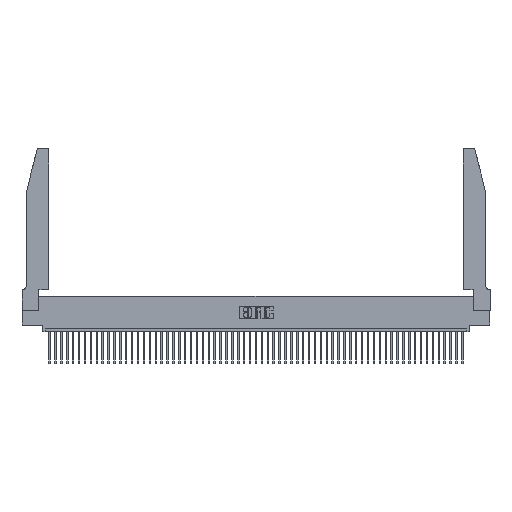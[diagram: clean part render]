
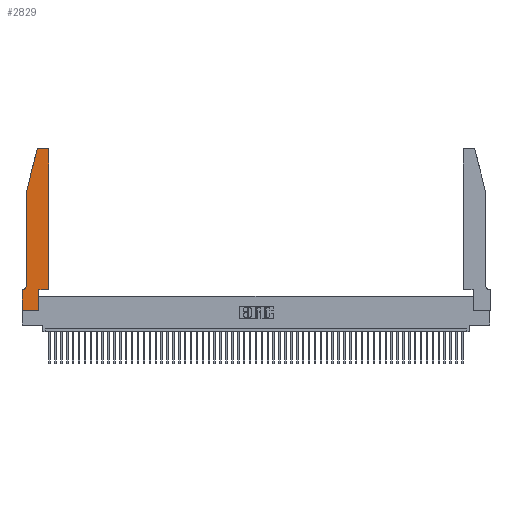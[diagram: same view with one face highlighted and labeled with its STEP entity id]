
A CAD part, top view. The second image highlights one B-rep face of the part: STEP entity #2829.
In plain terms, the highlighted planar face has unit normal (0, 0, 1).
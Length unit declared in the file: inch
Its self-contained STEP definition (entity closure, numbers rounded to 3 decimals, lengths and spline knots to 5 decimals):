
#566 = EDGE_CURVE ( 'NONE', #36919, #50856, #39967, .T. ) ;
#1370 = CARTESIAN_POINT ( 'NONE',  ( 0.284, 2.72, 0.37 ) ) ;
#1416 = CARTESIAN_POINT ( 'NONE',  ( 0.2865, 0.35, 0.37 ) ) ;
#1967 = VERTEX_POINT ( 'NONE', #28017 ) ;
#2055 = DIRECTION ( 'NONE',  ( 0., 0., 1. ) ) ;
#2248 = ORIENTED_EDGE ( 'NONE', *, *, #53547, .T. ) ;
#2305 = DIRECTION ( 'NONE',  ( 0., 1., 0. ) ) ;
#2829 = ADVANCED_FACE ( 'NONE', ( #20331 ), #9238, .T. ) ;
#3087 = EDGE_CURVE ( 'NONE', #14499, #12628, #45249, .T. ) ;
#3220 = CARTESIAN_POINT ( 'NONE',  ( 0.0755, 0.35, 0.37 ) ) ;
#4333 = CARTESIAN_POINT ( 'NONE',  ( 0.4505, 0.35, 0.37 ) ) ;
#5033 = VECTOR ( 'NONE', #30025, 39.37008 ) ;
#5666 = VERTEX_POINT ( 'NONE', #31880 ) ;
#5873 = LINE ( 'NONE', #32470, #36101 ) ;
#6248 = LINE ( 'NONE', #3220, #34407 ) ;
#7777 = AXIS2_PLACEMENT_3D ( 'NONE', #36329, #44796, #54358 ) ;
#8421 = AXIS2_PLACEMENT_3D ( 'NONE', #1370, #13735, #34801 ) ;
#8667 = CARTESIAN_POINT ( 'NONE',  ( 0.0055, 0.35, 0.37 ) ) ;
#8744 = ORIENTED_EDGE ( 'NONE', *, *, #42962, .T. ) ;
#9056 = DIRECTION ( 'NONE',  ( -0.239, -0.971, 0. ) ) ;
#9238 = PLANE ( 'NONE',  #32448 ) ;
#9537 = CIRCLE ( 'NONE', #7777, 0.07 ) ;
#9663 = VECTOR ( 'NONE', #33040, 39.37008 ) ;
#12628 = VERTEX_POINT ( 'NONE', #13793 ) ;
#13256 = CARTESIAN_POINT ( 'NONE',  ( 0.0755, 0.42, 0.37 ) ) ;
#13407 = DIRECTION ( 'NONE',  ( 0., 0., 1. ) ) ;
#13735 = DIRECTION ( 'NONE',  ( 0., 0., 1. ) ) ;
#13793 = CARTESIAN_POINT ( 'NONE',  ( 0.2865, 0., 0.37 ) ) ;
#14499 = VERTEX_POINT ( 'NONE', #18149 ) ;
#15003 = VERTEX_POINT ( 'NONE', #18124 ) ;
#16359 = VECTOR ( 'NONE', #44993, 39.37008 ) ;
#16965 = DIRECTION ( 'NONE',  ( 1., 0., 0. ) ) ;
#18124 = CARTESIAN_POINT ( 'NONE',  ( 0.25487, 2.72718, 0.37 ) ) ;
#18149 = CARTESIAN_POINT ( 'NONE',  ( 0., 0., 0.37 ) ) ;
#19141 = CARTESIAN_POINT ( 'NONE',  ( 0.4205, 2.75, 0.37 ) ) ;
#19501 = ORIENTED_EDGE ( 'NONE', *, *, #33910, .T. ) ;
#20331 = FACE_OUTER_BOUND ( 'NONE', #47526, .T. ) ;
#20397 = VERTEX_POINT ( 'NONE', #1416 ) ;
#20474 = VERTEX_POINT ( 'NONE', #39636 ) ;
#21103 = LINE ( 'NONE', #50409, #49385 ) ;
#23500 = AXIS2_PLACEMENT_3D ( 'NONE', #41394, #13407, #16965 ) ;
#24603 = ORIENTED_EDGE ( 'NONE', *, *, #41780, .T. ) ;
#26401 = VERTEX_POINT ( 'NONE', #13256 ) ;
#27367 = LINE ( 'NONE', #31984, #51041 ) ;
#27885 = DIRECTION ( 'NONE',  ( -1., 0., 0. ) ) ;
#28017 = CARTESIAN_POINT ( 'NONE',  ( 0.4505, 2.72, 0.37 ) ) ;
#28626 = ORIENTED_EDGE ( 'NONE', *, *, #3087, .T. ) ;
#29058 = LINE ( 'NONE', #35685, #40902 ) ;
#29321 = EDGE_CURVE ( 'NONE', #15003, #5666, #21103, .T. ) ;
#30025 = DIRECTION ( 'NONE',  ( 1., 0., 0. ) ) ;
#30283 = CARTESIAN_POINT ( 'NONE',  ( 0., 0.35, 0.37 ) ) ;
#31880 = CARTESIAN_POINT ( 'NONE',  ( 0.0755, 2., 0.37 ) ) ;
#31984 = CARTESIAN_POINT ( 'NONE',  ( 0.0755, 2., 0.37 ) ) ;
#32448 = AXIS2_PLACEMENT_3D ( 'NONE', #30283, #2055, #47772 ) ;
#32470 = CARTESIAN_POINT ( 'NONE',  ( 0.4505, 0.35, 0.37 ) ) ;
#33040 = DIRECTION ( 'NONE',  ( 0., -1., 0. ) ) ;
#33208 = ORIENTED_EDGE ( 'NONE', *, *, #36933, .T. ) ;
#33346 = LINE ( 'NONE', #36928, #9663 ) ;
#33910 = EDGE_CURVE ( 'NONE', #12628, #20397, #29058, .T. ) ;
#34407 = VECTOR ( 'NONE', #41212, 39.37008 ) ;
#34801 = DIRECTION ( 'NONE',  ( 1., 0., 0. ) ) ;
#35309 = CARTESIAN_POINT ( 'NONE',  ( 0.4505, 0.35, 0.37 ) ) ;
#35685 = CARTESIAN_POINT ( 'NONE',  ( 0.2865, 0.35, 0.37 ) ) ;
#35708 = ORIENTED_EDGE ( 'NONE', *, *, #29321, .T. ) ;
#36101 = VECTOR ( 'NONE', #36720, 39.37008 ) ;
#36329 = CARTESIAN_POINT ( 'NONE',  ( 0.0055, 0.42, 0.37 ) ) ;
#36484 = CARTESIAN_POINT ( 'NONE',  ( 0.284, 2.75, 0.37 ) ) ;
#36720 = DIRECTION ( 'NONE',  ( 0., 1., 0. ) ) ;
#36919 = VERTEX_POINT ( 'NONE', #19141 ) ;
#36928 = CARTESIAN_POINT ( 'NONE',  ( 0., 0., 0.37 ) ) ;
#36933 = EDGE_CURVE ( 'NONE', #5666, #26401, #27367, .T. ) ;
#37099 = EDGE_CURVE ( 'NONE', #20397, #39069, #38512, .T. ) ;
#37737 = ORIENTED_EDGE ( 'NONE', *, *, #38920, .T. ) ;
#38091 = ORIENTED_EDGE ( 'NONE', *, *, #51934, .T. ) ;
#38512 = LINE ( 'NONE', #35309, #5033 ) ;
#38880 = DIRECTION ( 'NONE',  ( 0., -1., 0. ) ) ;
#38920 = EDGE_CURVE ( 'NONE', #41231, #20474, #6248, .T. ) ;
#39069 = VERTEX_POINT ( 'NONE', #4333 ) ;
#39636 = CARTESIAN_POINT ( 'NONE',  ( 0., 0.35, 0.37 ) ) ;
#39967 = LINE ( 'NONE', #48871, #46569 ) ;
#40902 = VECTOR ( 'NONE', #2305, 39.37008 ) ;
#41212 = DIRECTION ( 'NONE',  ( -1., 0., 0. ) ) ;
#41231 = VERTEX_POINT ( 'NONE', #8667 ) ;
#41394 = CARTESIAN_POINT ( 'NONE',  ( 0.4205, 2.72, 0.37 ) ) ;
#41780 = EDGE_CURVE ( 'NONE', #39069, #1967, #5873, .T. ) ;
#42962 = EDGE_CURVE ( 'NONE', #1967, #36919, #44549, .T. ) ;
#44506 = EDGE_CURVE ( 'NONE', #26401, #41231, #9537, .T. ) ;
#44549 = CIRCLE ( 'NONE', #23500, 0.03 ) ;
#44796 = DIRECTION ( 'NONE',  ( 0., 0., -1. ) ) ;
#44993 = DIRECTION ( 'NONE',  ( 1., 0., 0. ) ) ;
#45183 = CARTESIAN_POINT ( 'NONE',  ( 0., 0., 0.37 ) ) ;
#45249 = LINE ( 'NONE', #45183, #16359 ) ;
#46569 = VECTOR ( 'NONE', #27885, 39.37008 ) ;
#47526 = EDGE_LOOP ( 'NONE', ( #50729, #2248, #35708, #33208, #52988, #37737, #38091, #28626, #19501, #50051, #24603, #8744 ) ) ;
#47772 = DIRECTION ( 'NONE',  ( 1., 0., 0. ) ) ;
#48871 = CARTESIAN_POINT ( 'NONE',  ( 0.2605, 2.75, 0.37 ) ) ;
#49385 = VECTOR ( 'NONE', #9056, 39.37008 ) ;
#50051 = ORIENTED_EDGE ( 'NONE', *, *, #37099, .T. ) ;
#50409 = CARTESIAN_POINT ( 'NONE',  ( 0.0755, 2., 0.37 ) ) ;
#50729 = ORIENTED_EDGE ( 'NONE', *, *, #566, .T. ) ;
#50856 = VERTEX_POINT ( 'NONE', #36484 ) ;
#50924 = CIRCLE ( 'NONE', #8421, 0.03 ) ;
#51041 = VECTOR ( 'NONE', #38880, 39.37008 ) ;
#51934 = EDGE_CURVE ( 'NONE', #20474, #14499, #33346, .T. ) ;
#52988 = ORIENTED_EDGE ( 'NONE', *, *, #44506, .T. ) ;
#53547 = EDGE_CURVE ( 'NONE', #50856, #15003, #50924, .T. ) ;
#54358 = DIRECTION ( 'NONE',  ( -1., 0., 0. ) ) ;
